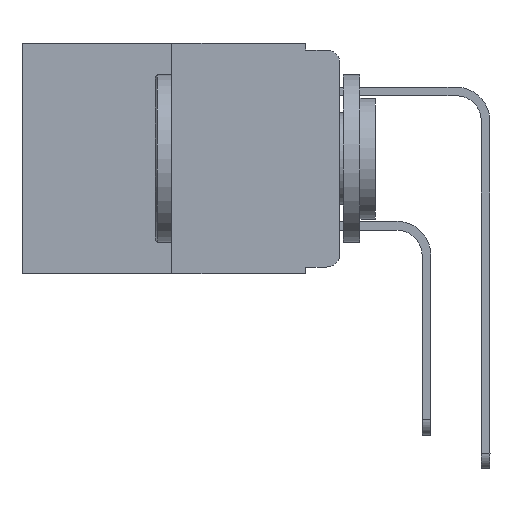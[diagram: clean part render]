
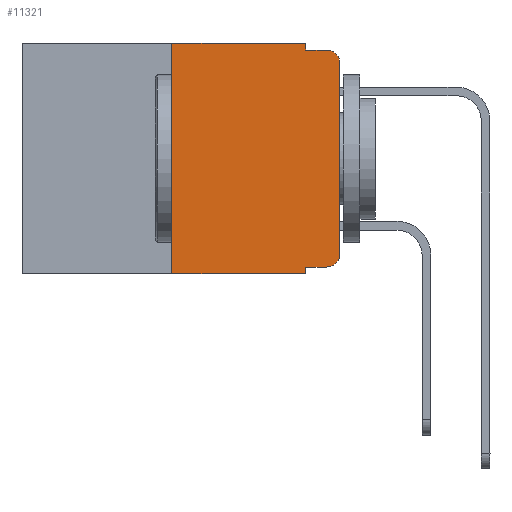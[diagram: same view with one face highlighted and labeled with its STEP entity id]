
A CAD part, left-side view. The second image highlights one B-rep face of the part: STEP entity #11321.
In plain terms, the highlighted planar face has unit normal (-1, 0, 0).
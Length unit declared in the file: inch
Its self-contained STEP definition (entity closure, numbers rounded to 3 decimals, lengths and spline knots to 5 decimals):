
#471 = ORIENTED_EDGE ( 'NONE', *, *, #20529, .T. ) ;
#1160 = VERTEX_POINT ( 'NONE', #18660 ) ;
#1705 = VERTEX_POINT ( 'NONE', #19991 ) ;
#2963 = VERTEX_POINT ( 'NONE', #14890 ) ;
#3250 = VECTOR ( 'NONE', #7873, 39.37008 ) ;
#4690 = VECTOR ( 'NONE', #22091, 39.37008 ) ;
#4886 = VERTEX_POINT ( 'NONE', #19839 ) ;
#5123 = CARTESIAN_POINT ( 'NONE',  ( 0., 0.051, 0. ) ) ;
#5582 = CARTESIAN_POINT ( 'NONE',  ( 0., 0., -0.03 ) ) ;
#5645 = CARTESIAN_POINT ( 'NONE',  ( 0., 0.02, -0.03 ) ) ;
#5895 = DIRECTION ( 'NONE',  ( -1., 0., 0. ) ) ;
#6128 = VECTOR ( 'NONE', #7345, 39.37008 ) ;
#6463 = VERTEX_POINT ( 'NONE', #14583 ) ;
#6581 = VECTOR ( 'NONE', #10561, 39.37008 ) ;
#6660 = VECTOR ( 'NONE', #13423, 39.37008 ) ;
#6741 = EDGE_LOOP ( 'NONE', ( #13403, #17543, #18426, #17820, #20000, #9610, #471, #26150, #12155, #14933 ) ) ;
#7060 = EDGE_CURVE ( 'NONE', #4886, #1160, #9831, .T. ) ;
#7162 = CIRCLE ( 'NONE', #18187, 0.02 ) ;
#7345 = DIRECTION ( 'NONE',  ( 0., 0., 1. ) ) ;
#7693 = PLANE ( 'NONE',  #15034 ) ;
#7873 = DIRECTION ( 'NONE',  ( 0., -1., 0. ) ) ;
#8101 = CARTESIAN_POINT ( 'NONE',  ( 0., 0.25, -0.343 ) ) ;
#8993 = VERTEX_POINT ( 'NONE', #10526 ) ;
#9395 = LINE ( 'NONE', #17837, #6660 ) ;
#9580 = DIRECTION ( 'NONE',  ( 1., 0., 0. ) ) ;
#9610 = ORIENTED_EDGE ( 'NONE', *, *, #28123, .F. ) ;
#9831 = LINE ( 'NONE', #18567, #18751 ) ;
#9974 = DIRECTION ( 'NONE',  ( 0., 0., -1. ) ) ;
#10131 = EDGE_CURVE ( 'NONE', #2963, #1705, #7162, .T. ) ;
#10526 = CARTESIAN_POINT ( 'NONE',  ( 0., 0.051, -0.01 ) ) ;
#10561 = DIRECTION ( 'NONE',  ( 0., 0., 1. ) ) ;
#10578 = VERTEX_POINT ( 'NONE', #5582 ) ;
#11238 = CARTESIAN_POINT ( 'NONE',  ( 0., 0.473, 0. ) ) ;
#11321 = ADVANCED_FACE ( 'NONE', ( #12024 ), #7693, .F. ) ;
#11901 = LINE ( 'NONE', #5123, #21040 ) ;
#12024 = FACE_OUTER_BOUND ( 'NONE', #6741, .T. ) ;
#12145 = AXIS2_PLACEMENT_3D ( 'NONE', #5645, #27769, #25467 ) ;
#12155 = ORIENTED_EDGE ( 'NONE', *, *, #15326, .T. ) ;
#12388 = CARTESIAN_POINT ( 'NONE',  ( 0., 0.02, -0.313 ) ) ;
#13199 = VERTEX_POINT ( 'NONE', #8101 ) ;
#13403 = ORIENTED_EDGE ( 'NONE', *, *, #27793, .T. ) ;
#13423 = DIRECTION ( 'NONE',  ( 0., -1., 0. ) ) ;
#13920 = DIRECTION ( 'NONE',  ( 0., 0., -1. ) ) ;
#14430 = CARTESIAN_POINT ( 'NONE',  ( 0., 0.051, -0.01 ) ) ;
#14539 = CARTESIAN_POINT ( 'NONE',  ( 0., 0.051, 0. ) ) ;
#14583 = CARTESIAN_POINT ( 'NONE',  ( 0., 0.25, 0. ) ) ;
#14890 = CARTESIAN_POINT ( 'NONE',  ( 0., 0.02, -0.333 ) ) ;
#14933 = ORIENTED_EDGE ( 'NONE', *, *, #10131, .T. ) ;
#15034 = AXIS2_PLACEMENT_3D ( 'NONE', #18595, #9580, #23171 ) ;
#15130 = CARTESIAN_POINT ( 'NONE',  ( 0., 0., 0. ) ) ;
#15326 = EDGE_CURVE ( 'NONE', #4886, #2963, #20914, .T. ) ;
#16625 = CARTESIAN_POINT ( 'NONE',  ( 0., 0.02, -0.01 ) ) ;
#16704 = DIRECTION ( 'NONE',  ( 0., -1., 0. ) ) ;
#17543 = ORIENTED_EDGE ( 'NONE', *, *, #20192, .T. ) ;
#17820 = ORIENTED_EDGE ( 'NONE', *, *, #22837, .F. ) ;
#17837 = CARTESIAN_POINT ( 'NONE',  ( 0., 0.473, -0.343 ) ) ;
#18092 = EDGE_CURVE ( 'NONE', #6463, #22019, #20346, .T. ) ;
#18187 = AXIS2_PLACEMENT_3D ( 'NONE', #12388, #5895, #18819 ) ;
#18426 = ORIENTED_EDGE ( 'NONE', *, *, #20168, .F. ) ;
#18567 = CARTESIAN_POINT ( 'NONE',  ( 0., 0.051, 0. ) ) ;
#18595 = CARTESIAN_POINT ( 'NONE',  ( 0., 0.473, 0. ) ) ;
#18660 = CARTESIAN_POINT ( 'NONE',  ( 0., 0.051, -0.343 ) ) ;
#18751 = VECTOR ( 'NONE', #9974, 39.37008 ) ;
#18819 = DIRECTION ( 'NONE',  ( 0., 0., -1. ) ) ;
#19270 = LINE ( 'NONE', #15130, #6581 ) ;
#19839 = CARTESIAN_POINT ( 'NONE',  ( 0., 0.051, -0.333 ) ) ;
#19991 = CARTESIAN_POINT ( 'NONE',  ( 0., 0., -0.313 ) ) ;
#20000 = ORIENTED_EDGE ( 'NONE', *, *, #18092, .F. ) ;
#20168 = EDGE_CURVE ( 'NONE', #8993, #27532, #27341, .T. ) ;
#20192 = EDGE_CURVE ( 'NONE', #10578, #27532, #24503, .T. ) ;
#20346 = LINE ( 'NONE', #11238, #4690 ) ;
#20529 = EDGE_CURVE ( 'NONE', #13199, #1160, #9395, .T. ) ;
#20914 = LINE ( 'NONE', #23346, #3250 ) ;
#21040 = VECTOR ( 'NONE', #13920, 39.37008 ) ;
#22019 = VERTEX_POINT ( 'NONE', #14539 ) ;
#22091 = DIRECTION ( 'NONE',  ( 0., -1., 0. ) ) ;
#22691 = CARTESIAN_POINT ( 'NONE',  ( 0., 0.25, 0. ) ) ;
#22837 = EDGE_CURVE ( 'NONE', #22019, #8993, #11901, .T. ) ;
#22971 = LINE ( 'NONE', #22691, #6128 ) ;
#23171 = DIRECTION ( 'NONE',  ( 0., 0., -1. ) ) ;
#23346 = CARTESIAN_POINT ( 'NONE',  ( 0., 0.051, -0.333 ) ) ;
#24503 = CIRCLE ( 'NONE', #12145, 0.02 ) ;
#25467 = DIRECTION ( 'NONE',  ( 0., 0., -1. ) ) ;
#26150 = ORIENTED_EDGE ( 'NONE', *, *, #7060, .F. ) ;
#27341 = LINE ( 'NONE', #14430, #28188 ) ;
#27532 = VERTEX_POINT ( 'NONE', #16625 ) ;
#27769 = DIRECTION ( 'NONE',  ( -1., 0., 0. ) ) ;
#27793 = EDGE_CURVE ( 'NONE', #1705, #10578, #19270, .T. ) ;
#28123 = EDGE_CURVE ( 'NONE', #13199, #6463, #22971, .T. ) ;
#28188 = VECTOR ( 'NONE', #16704, 39.37008 ) ;
